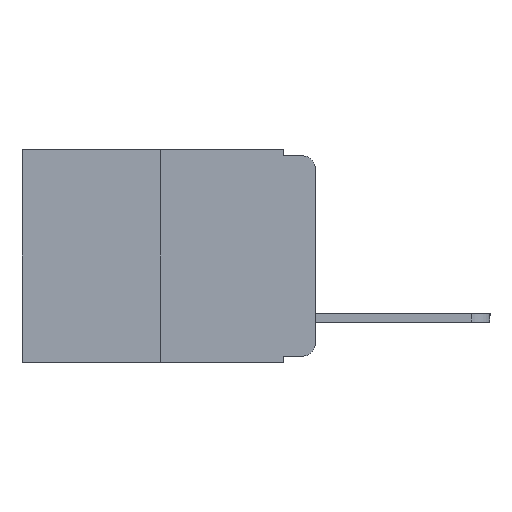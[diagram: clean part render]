
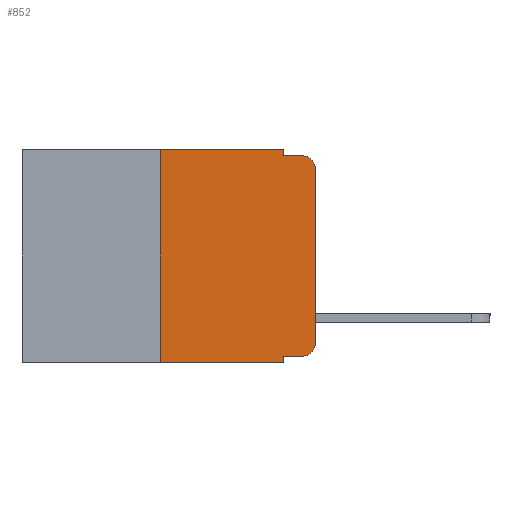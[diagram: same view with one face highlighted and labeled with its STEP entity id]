
A CAD part, left-side view. The second image highlights one B-rep face of the part: STEP entity #852.
In plain terms, the highlighted planar face has unit normal (-1, 0, 0).
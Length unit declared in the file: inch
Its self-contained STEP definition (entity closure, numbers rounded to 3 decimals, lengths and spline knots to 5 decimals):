
#129 = CARTESIAN_POINT ( 'NONE',  ( 0., 0.02, -0.333 ) ) ;
#154 = LINE ( 'NONE', #6123, #11779 ) ;
#161 = ORIENTED_EDGE ( 'NONE', *, *, #12599, .T. ) ;
#250 = DIRECTION ( 'NONE',  ( 0., -1., 0. ) ) ;
#290 = DIRECTION ( 'NONE',  ( 0., 0., 1. ) ) ;
#483 = ORIENTED_EDGE ( 'NONE', *, *, #8912, .F. ) ;
#852 = ADVANCED_FACE ( 'NONE', ( #4535 ), #1929, .F. ) ;
#865 = CARTESIAN_POINT ( 'NONE',  ( 0., 0.02, -0.03 ) ) ;
#887 = ORIENTED_EDGE ( 'NONE', *, *, #7448, .F. ) ;
#1645 = VERTEX_POINT ( 'NONE', #13603 ) ;
#1929 = PLANE ( 'NONE',  #3293 ) ;
#2040 = VERTEX_POINT ( 'NONE', #12824 ) ;
#2190 = DIRECTION ( 'NONE',  ( 0., 0., -1. ) ) ;
#2716 = VERTEX_POINT ( 'NONE', #5110 ) ;
#2794 = VECTOR ( 'NONE', #9764, 39.37008 ) ;
#2833 = VECTOR ( 'NONE', #4922, 39.37008 ) ;
#3293 = AXIS2_PLACEMENT_3D ( 'NONE', #5467, #13230, #13016 ) ;
#3352 = DIRECTION ( 'NONE',  ( -1., 0., 0. ) ) ;
#3812 = CARTESIAN_POINT ( 'NONE',  ( 0., 0.473, -0.343 ) ) ;
#3860 = CARTESIAN_POINT ( 'NONE',  ( 0., 0.051, 0. ) ) ;
#4184 = ORIENTED_EDGE ( 'NONE', *, *, #13372, .F. ) ;
#4222 = CARTESIAN_POINT ( 'NONE',  ( 0., 0.02, -0.01 ) ) ;
#4535 = FACE_OUTER_BOUND ( 'NONE', #7503, .T. ) ;
#4611 = DIRECTION ( 'NONE',  ( 0., -1., 0. ) ) ;
#4922 = DIRECTION ( 'NONE',  ( 0., -1., 0. ) ) ;
#5060 = CARTESIAN_POINT ( 'NONE',  ( 0., 0., 0. ) ) ;
#5110 = CARTESIAN_POINT ( 'NONE',  ( 0., 0.25, -0.343 ) ) ;
#5426 = VECTOR ( 'NONE', #13527, 39.37008 ) ;
#5467 = CARTESIAN_POINT ( 'NONE',  ( 0., 0.473, 0. ) ) ;
#5805 = LINE ( 'NONE', #3812, #2833 ) ;
#5874 = ORIENTED_EDGE ( 'NONE', *, *, #12686, .T. ) ;
#5936 = CARTESIAN_POINT ( 'NONE',  ( 0., 0.051, 0. ) ) ;
#5981 = EDGE_CURVE ( 'NONE', #2716, #8318, #9004, .T. ) ;
#6123 = CARTESIAN_POINT ( 'NONE',  ( 0., 0.473, 0. ) ) ;
#6502 = CIRCLE ( 'NONE', #12763, 0.02 ) ;
#6858 = CARTESIAN_POINT ( 'NONE',  ( 0., 0.051, -0.01 ) ) ;
#7037 = DIRECTION ( 'NONE',  ( 0., 0., -1. ) ) ;
#7448 = EDGE_CURVE ( 'NONE', #12637, #9835, #11173, .T. ) ;
#7503 = EDGE_LOOP ( 'NONE', ( #13500, #11105, #483, #887, #13660, #11119, #161, #4184, #5874, #13557 ) ) ;
#7516 = VECTOR ( 'NONE', #290, 39.37008 ) ;
#7771 = LINE ( 'NONE', #7870, #13056 ) ;
#7870 = CARTESIAN_POINT ( 'NONE',  ( 0., 0.051, -0.01 ) ) ;
#8219 = VERTEX_POINT ( 'NONE', #129 ) ;
#8318 = VERTEX_POINT ( 'NONE', #12507 ) ;
#8657 = CARTESIAN_POINT ( 'NONE',  ( 0., 0.25, 0. ) ) ;
#8847 = DIRECTION ( 'NONE',  ( -1., 0., 0. ) ) ;
#8912 = EDGE_CURVE ( 'NONE', #9835, #9431, #7771, .T. ) ;
#9004 = LINE ( 'NONE', #8657, #2794 ) ;
#9431 = VERTEX_POINT ( 'NONE', #4222 ) ;
#9764 = DIRECTION ( 'NONE',  ( 0., 0., 1. ) ) ;
#9835 = VERTEX_POINT ( 'NONE', #6858 ) ;
#9911 = CARTESIAN_POINT ( 'NONE',  ( 0., 0.02, -0.313 ) ) ;
#10117 = EDGE_CURVE ( 'NONE', #8318, #12637, #154, .T. ) ;
#10207 = CARTESIAN_POINT ( 'NONE',  ( 0., 0., -0.03 ) ) ;
#10370 = EDGE_CURVE ( 'NONE', #11459, #9431, #12531, .T. ) ;
#10410 = LINE ( 'NONE', #5060, #7516 ) ;
#10429 = CARTESIAN_POINT ( 'NONE',  ( 0., 0.051, 0. ) ) ;
#10794 = VERTEX_POINT ( 'NONE', #11520 ) ;
#10899 = LINE ( 'NONE', #13535, #13611 ) ;
#10987 = DIRECTION ( 'NONE',  ( 0., 0., -1. ) ) ;
#11105 = ORIENTED_EDGE ( 'NONE', *, *, #10370, .T. ) ;
#11119 = ORIENTED_EDGE ( 'NONE', *, *, #5981, .F. ) ;
#11173 = LINE ( 'NONE', #10429, #5426 ) ;
#11459 = VERTEX_POINT ( 'NONE', #10207 ) ;
#11520 = CARTESIAN_POINT ( 'NONE',  ( 0., 0., -0.313 ) ) ;
#11532 = DIRECTION ( 'NONE',  ( 0., -1., 0. ) ) ;
#11779 = VECTOR ( 'NONE', #11532, 39.37008 ) ;
#12014 = EDGE_CURVE ( 'NONE', #8219, #10794, #6502, .T. ) ;
#12025 = VECTOR ( 'NONE', #7037, 39.37008 ) ;
#12427 = EDGE_CURVE ( 'NONE', #10794, #11459, #10410, .T. ) ;
#12507 = CARTESIAN_POINT ( 'NONE',  ( 0., 0.25, 0. ) ) ;
#12531 = CIRCLE ( 'NONE', #12575, 0.02 ) ;
#12575 = AXIS2_PLACEMENT_3D ( 'NONE', #865, #8847, #2190 ) ;
#12599 = EDGE_CURVE ( 'NONE', #2716, #2040, #5805, .T. ) ;
#12637 = VERTEX_POINT ( 'NONE', #3860 ) ;
#12686 = EDGE_CURVE ( 'NONE', #1645, #8219, #10899, .T. ) ;
#12763 = AXIS2_PLACEMENT_3D ( 'NONE', #9911, #3352, #10987 ) ;
#12824 = CARTESIAN_POINT ( 'NONE',  ( 0., 0.051, -0.343 ) ) ;
#13016 = DIRECTION ( 'NONE',  ( 0., 0., -1. ) ) ;
#13056 = VECTOR ( 'NONE', #4611, 39.37008 ) ;
#13230 = DIRECTION ( 'NONE',  ( 1., 0., 0. ) ) ;
#13372 = EDGE_CURVE ( 'NONE', #1645, #2040, #13772, .T. ) ;
#13500 = ORIENTED_EDGE ( 'NONE', *, *, #12427, .T. ) ;
#13527 = DIRECTION ( 'NONE',  ( 0., 0., -1. ) ) ;
#13535 = CARTESIAN_POINT ( 'NONE',  ( 0., 0.051, -0.333 ) ) ;
#13557 = ORIENTED_EDGE ( 'NONE', *, *, #12014, .T. ) ;
#13603 = CARTESIAN_POINT ( 'NONE',  ( 0., 0.051, -0.333 ) ) ;
#13611 = VECTOR ( 'NONE', #250, 39.37008 ) ;
#13660 = ORIENTED_EDGE ( 'NONE', *, *, #10117, .F. ) ;
#13772 = LINE ( 'NONE', #5936, #12025 ) ;
